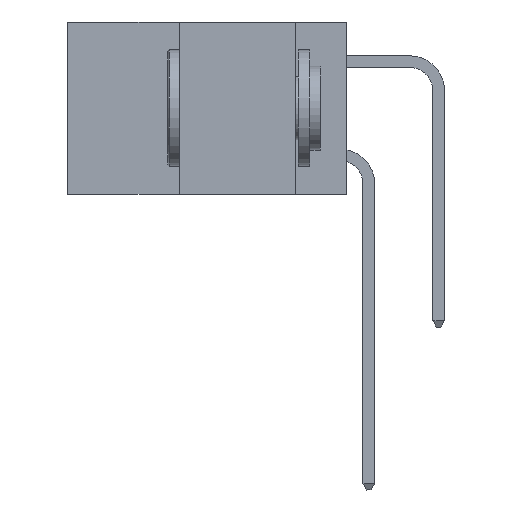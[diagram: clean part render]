
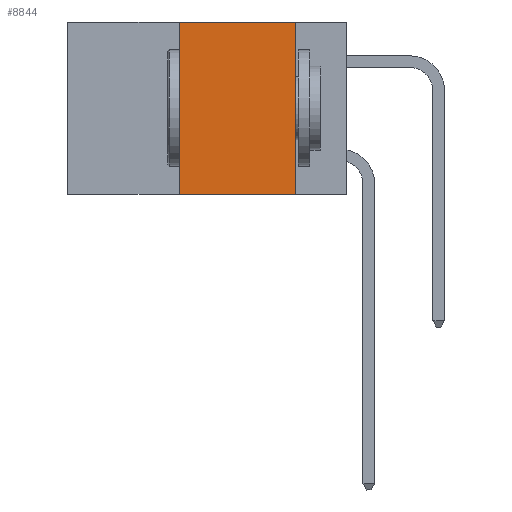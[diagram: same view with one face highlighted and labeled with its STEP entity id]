
A CAD part, left-side view. The second image highlights one B-rep face of the part: STEP entity #8844.
In plain terms, the highlighted planar face has unit normal (-1, 0, 0).
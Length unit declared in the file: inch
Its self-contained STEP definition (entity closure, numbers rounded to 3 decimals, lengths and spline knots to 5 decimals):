
#787 = CARTESIAN_POINT ( 'NONE',  ( 0., 0.36, 0. ) ) ;
#1229 = PLANE ( 'NONE',  #9424 ) ;
#1641 = VECTOR ( 'NONE', #2727, 39.37008 ) ;
#1663 = LINE ( 'NONE', #8723, #4086 ) ;
#1784 = VERTEX_POINT ( 'NONE', #7023 ) ;
#2202 = DIRECTION ( 'NONE',  ( 0., 0., -1. ) ) ;
#2274 = DIRECTION ( 'NONE',  ( 0., -1., 0. ) ) ;
#2655 = CARTESIAN_POINT ( 'NONE',  ( 0., 0.36, 0. ) ) ;
#2727 = DIRECTION ( 'NONE',  ( 0., 0., 1. ) ) ;
#2982 = VECTOR ( 'NONE', #2274, 39.37008 ) ;
#3085 = VERTEX_POINT ( 'NONE', #4204 ) ;
#3207 = CARTESIAN_POINT ( 'NONE',  ( 0., 0.6, -0.37 ) ) ;
#3438 = EDGE_CURVE ( 'NONE', #10749, #3085, #1663, .T. ) ;
#3749 = ORIENTED_EDGE ( 'NONE', *, *, #3438, .F. ) ;
#4071 = LINE ( 'NONE', #7945, #8677 ) ;
#4086 = VECTOR ( 'NONE', #8678, 39.37008 ) ;
#4204 = CARTESIAN_POINT ( 'NONE',  ( 0., 0.11, 0. ) ) ;
#4395 = EDGE_CURVE ( 'NONE', #1784, #10749, #6398, .T. ) ;
#4485 = EDGE_LOOP ( 'NONE', ( #8077, #3749, #8335, #6348 ) ) ;
#5341 = LINE ( 'NONE', #3207, #2982 ) ;
#6052 = CARTESIAN_POINT ( 'NONE',  ( 0., 0.11, -0.37 ) ) ;
#6348 = ORIENTED_EDGE ( 'NONE', *, *, #7505, .T. ) ;
#6398 = LINE ( 'NONE', #2655, #1641 ) ;
#7023 = CARTESIAN_POINT ( 'NONE',  ( 0., 0.36, -0.37 ) ) ;
#7474 = DIRECTION ( 'NONE',  ( 1., 0., 0. ) ) ;
#7505 = EDGE_CURVE ( 'NONE', #1784, #9080, #5341, .T. ) ;
#7865 = EDGE_CURVE ( 'NONE', #3085, #9080, #4071, .T. ) ;
#7945 = CARTESIAN_POINT ( 'NONE',  ( 0., 0.11, 0. ) ) ;
#8077 = ORIENTED_EDGE ( 'NONE', *, *, #7865, .F. ) ;
#8335 = ORIENTED_EDGE ( 'NONE', *, *, #4395, .F. ) ;
#8677 = VECTOR ( 'NONE', #8805, 39.37008 ) ;
#8678 = DIRECTION ( 'NONE',  ( 0., -1., 0. ) ) ;
#8723 = CARTESIAN_POINT ( 'NONE',  ( 0., 0.6, 0. ) ) ;
#8805 = DIRECTION ( 'NONE',  ( 0., 0., -1. ) ) ;
#8844 = ADVANCED_FACE ( 'NONE', ( #11104 ), #1229, .F. ) ;
#9080 = VERTEX_POINT ( 'NONE', #6052 ) ;
#9424 = AXIS2_PLACEMENT_3D ( 'NONE', #10002, #7474, #2202 ) ;
#10002 = CARTESIAN_POINT ( 'NONE',  ( 0., 0.6, 0. ) ) ;
#10749 = VERTEX_POINT ( 'NONE', #787 ) ;
#11104 = FACE_OUTER_BOUND ( 'NONE', #4485, .T. ) ;
